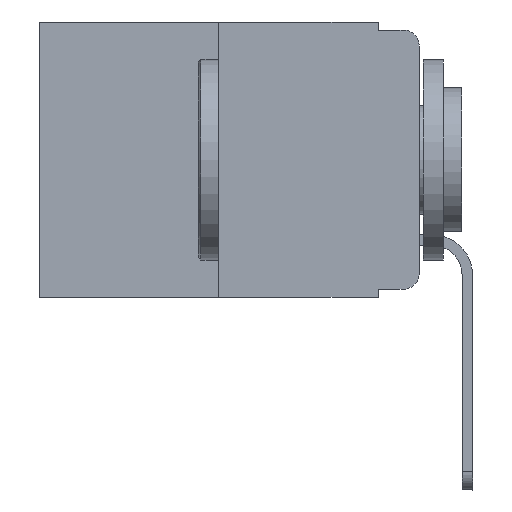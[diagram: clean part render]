
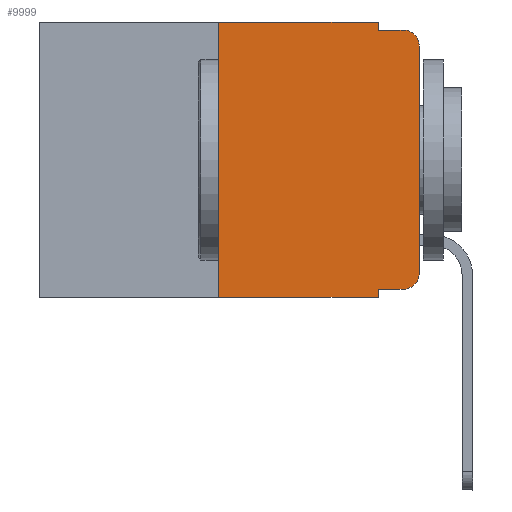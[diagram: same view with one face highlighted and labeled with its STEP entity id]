
A CAD part, left-side view. The second image highlights one B-rep face of the part: STEP entity #9999.
In plain terms, the highlighted planar face has unit normal (-1, 0, 0).
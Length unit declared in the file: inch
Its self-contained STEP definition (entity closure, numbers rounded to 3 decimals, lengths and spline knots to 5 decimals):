
#41 = DIRECTION ( 'NONE',  ( 0., 0., 1. ) ) ;
#108 = CARTESIAN_POINT ( 'NONE',  ( 0., 0.25, 0. ) ) ;
#129 = CARTESIAN_POINT ( 'NONE',  ( 0., 0.051, 0. ) ) ;
#133 = CARTESIAN_POINT ( 'NONE',  ( 0., 0.051, 0. ) ) ;
#196 = EDGE_LOOP ( 'NONE', ( #4954, #14652, #12975, #16622, #11611, #17615, #6983, #681, #12473, #16593 ) ) ;
#231 = DIRECTION ( 'NONE',  ( 0., 0., -1. ) ) ;
#298 = EDGE_CURVE ( 'NONE', #4578, #8122, #9774, .T. ) ;
#317 = AXIS2_PLACEMENT_3D ( 'NONE', #5507, #17931, #231 ) ;
#363 = EDGE_CURVE ( 'NONE', #11986, #3125, #1502, .T. ) ;
#462 = CARTESIAN_POINT ( 'NONE',  ( 0., 0.051, 0. ) ) ;
#677 = PLANE ( 'NONE',  #17012 ) ;
#681 = ORIENTED_EDGE ( 'NONE', *, *, #1542, .F. ) ;
#1209 = DIRECTION ( 'NONE',  ( 0., 0., 1. ) ) ;
#1366 = VECTOR ( 'NONE', #10932, 39.37008 ) ;
#1502 = LINE ( 'NONE', #133, #2758 ) ;
#1542 = EDGE_CURVE ( 'NONE', #6933, #9424, #12694, .T. ) ;
#1826 = DIRECTION ( 'NONE',  ( -1., 0., 0. ) ) ;
#1913 = DIRECTION ( 'NONE',  ( 0., 0., -1. ) ) ;
#1958 = EDGE_CURVE ( 'NONE', #15788, #9424, #7002, .T. ) ;
#2145 = CARTESIAN_POINT ( 'NONE',  ( 0., 0.473, 0. ) ) ;
#2154 = VECTOR ( 'NONE', #1209, 39.37008 ) ;
#2628 = EDGE_CURVE ( 'NONE', #3125, #12539, #9599, .T. ) ;
#2758 = VECTOR ( 'NONE', #5750, 39.37008 ) ;
#2809 = LINE ( 'NONE', #18081, #9546 ) ;
#2896 = DIRECTION ( 'NONE',  ( 0., -1., 0. ) ) ;
#3125 = VERTEX_POINT ( 'NONE', #15228 ) ;
#3644 = AXIS2_PLACEMENT_3D ( 'NONE', #4499, #1826, #1913 ) ;
#3800 = FACE_OUTER_BOUND ( 'NONE', #196, .T. ) ;
#4499 = CARTESIAN_POINT ( 'NONE',  ( 0., 0.02, -0.313 ) ) ;
#4578 = VERTEX_POINT ( 'NONE', #15416 ) ;
#4746 = CARTESIAN_POINT ( 'NONE',  ( 0., 0.25, 0. ) ) ;
#4954 = ORIENTED_EDGE ( 'NONE', *, *, #298, .T. ) ;
#5507 = CARTESIAN_POINT ( 'NONE',  ( 0., 0.02, -0.03 ) ) ;
#5639 = CARTESIAN_POINT ( 'NONE',  ( 0., 0.051, -0.333 ) ) ;
#5750 = DIRECTION ( 'NONE',  ( 0., 0., -1. ) ) ;
#6227 = CARTESIAN_POINT ( 'NONE',  ( 0., 0.02, -0.333 ) ) ;
#6259 = VERTEX_POINT ( 'NONE', #6227 ) ;
#6876 = CIRCLE ( 'NONE', #3644, 0.02 ) ;
#6933 = VERTEX_POINT ( 'NONE', #5639 ) ;
#6983 = ORIENTED_EDGE ( 'NONE', *, *, #1958, .T. ) ;
#7002 = LINE ( 'NONE', #17971, #1366 ) ;
#7075 = CIRCLE ( 'NONE', #317, 0.02 ) ;
#7144 = VECTOR ( 'NONE', #41, 39.37008 ) ;
#7325 = CARTESIAN_POINT ( 'NONE',  ( 0., 0.051, -0.343 ) ) ;
#7657 = DIRECTION ( 'NONE',  ( 1., 0., 0. ) ) ;
#8122 = VERTEX_POINT ( 'NONE', #9307 ) ;
#8245 = DIRECTION ( 'NONE',  ( 0., -1., 0. ) ) ;
#9128 = EDGE_CURVE ( 'NONE', #8122, #12539, #7075, .T. ) ;
#9141 = CARTESIAN_POINT ( 'NONE',  ( 0., 0.02, -0.01 ) ) ;
#9218 = EDGE_CURVE ( 'NONE', #17667, #11986, #12469, .T. ) ;
#9307 = CARTESIAN_POINT ( 'NONE',  ( 0., 0., -0.03 ) ) ;
#9424 = VERTEX_POINT ( 'NONE', #7325 ) ;
#9546 = VECTOR ( 'NONE', #2896, 39.37008 ) ;
#9599 = LINE ( 'NONE', #13783, #15503 ) ;
#9774 = LINE ( 'NONE', #15159, #7144 ) ;
#9999 = ADVANCED_FACE ( 'NONE', ( #3800 ), #677, .F. ) ;
#10714 = VECTOR ( 'NONE', #16794, 39.37008 ) ;
#10932 = DIRECTION ( 'NONE',  ( 0., -1., 0. ) ) ;
#11611 = ORIENTED_EDGE ( 'NONE', *, *, #9218, .F. ) ;
#11969 = DIRECTION ( 'NONE',  ( 0., -1., 0. ) ) ;
#11986 = VERTEX_POINT ( 'NONE', #462 ) ;
#12469 = LINE ( 'NONE', #15702, #15539 ) ;
#12473 = ORIENTED_EDGE ( 'NONE', *, *, #15937, .T. ) ;
#12539 = VERTEX_POINT ( 'NONE', #9141 ) ;
#12694 = LINE ( 'NONE', #129, #10714 ) ;
#12975 = ORIENTED_EDGE ( 'NONE', *, *, #2628, .F. ) ;
#13082 = EDGE_CURVE ( 'NONE', #15788, #17667, #13756, .T. ) ;
#13319 = DIRECTION ( 'NONE',  ( 0., 0., -1. ) ) ;
#13374 = EDGE_CURVE ( 'NONE', #6259, #4578, #6876, .T. ) ;
#13756 = LINE ( 'NONE', #108, #2154 ) ;
#13783 = CARTESIAN_POINT ( 'NONE',  ( 0., 0.051, -0.01 ) ) ;
#14529 = CARTESIAN_POINT ( 'NONE',  ( 0., 0.25, -0.343 ) ) ;
#14652 = ORIENTED_EDGE ( 'NONE', *, *, #9128, .T. ) ;
#15159 = CARTESIAN_POINT ( 'NONE',  ( 0., 0., 0. ) ) ;
#15228 = CARTESIAN_POINT ( 'NONE',  ( 0., 0.051, -0.01 ) ) ;
#15416 = CARTESIAN_POINT ( 'NONE',  ( 0., 0., -0.313 ) ) ;
#15503 = VECTOR ( 'NONE', #11969, 39.37008 ) ;
#15539 = VECTOR ( 'NONE', #8245, 39.37008 ) ;
#15702 = CARTESIAN_POINT ( 'NONE',  ( 0., 0.473, 0. ) ) ;
#15788 = VERTEX_POINT ( 'NONE', #14529 ) ;
#15937 = EDGE_CURVE ( 'NONE', #6933, #6259, #2809, .T. ) ;
#16593 = ORIENTED_EDGE ( 'NONE', *, *, #13374, .T. ) ;
#16622 = ORIENTED_EDGE ( 'NONE', *, *, #363, .F. ) ;
#16794 = DIRECTION ( 'NONE',  ( 0., 0., -1. ) ) ;
#17012 = AXIS2_PLACEMENT_3D ( 'NONE', #2145, #7657, #13319 ) ;
#17615 = ORIENTED_EDGE ( 'NONE', *, *, #13082, .F. ) ;
#17667 = VERTEX_POINT ( 'NONE', #4746 ) ;
#17931 = DIRECTION ( 'NONE',  ( -1., 0., 0. ) ) ;
#17971 = CARTESIAN_POINT ( 'NONE',  ( 0., 0.473, -0.343 ) ) ;
#18081 = CARTESIAN_POINT ( 'NONE',  ( 0., 0.051, -0.333 ) ) ;
